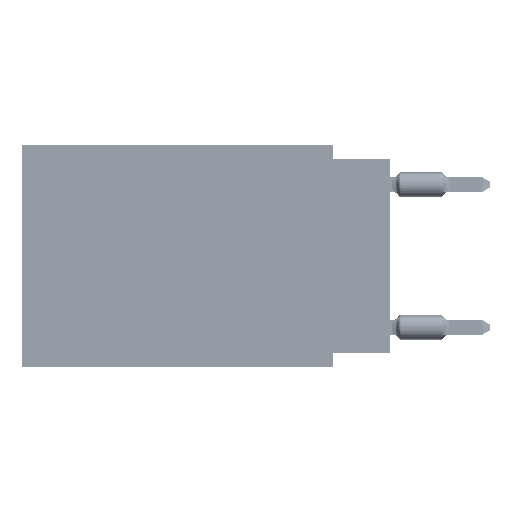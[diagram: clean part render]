
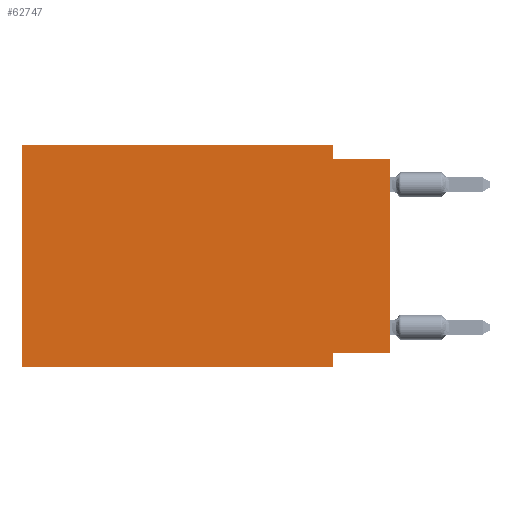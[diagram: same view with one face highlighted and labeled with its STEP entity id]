
A CAD part, left-side view. The second image highlights one B-rep face of the part: STEP entity #62747.
In plain terms, the highlighted planar face has unit normal (-1, 0, 0).
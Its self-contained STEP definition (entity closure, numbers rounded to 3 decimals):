
#709 = DIRECTION ( 'NONE',  ( 0., 0., -1. ) ) ;
#745 = LINE ( 'NONE', #27588, #38852 ) ;
#2618 = LINE ( 'NONE', #15208, #77627 ) ;
#3308 = EDGE_CURVE ( 'NONE', #63452, #78809, #53112, .T. ) ;
#4547 = VERTEX_POINT ( 'NONE', #11266 ) ;
#5590 = CARTESIAN_POINT ( 'NONE',  ( 0., 2.54, -9.271 ) ) ;
#5610 = EDGE_CURVE ( 'NONE', #64251, #78809, #2618, .T. ) ;
#5797 = VECTOR ( 'NONE', #46315, 1000. ) ;
#5839 = VERTEX_POINT ( 'NONE', #65967 ) ;
#6373 = VECTOR ( 'NONE', #71645, 1000. ) ;
#7146 = CARTESIAN_POINT ( 'NONE',  ( 0., 0., -0.635 ) ) ;
#11266 = CARTESIAN_POINT ( 'NONE',  ( 0., 2.54, -0.635 ) ) ;
#14900 = CARTESIAN_POINT ( 'NONE',  ( 0., 0., 0. ) ) ;
#15208 = CARTESIAN_POINT ( 'NONE',  ( 0., 16.383, -9.906 ) ) ;
#16245 = EDGE_CURVE ( 'NONE', #64251, #56325, #36313, .T. ) ;
#16995 = ORIENTED_EDGE ( 'NONE', *, *, #64843, .F. ) ;
#17209 = CARTESIAN_POINT ( 'NONE',  ( 0., 0., -9.271 ) ) ;
#17852 = EDGE_CURVE ( 'NONE', #73377, #50432, #28324, .T. ) ;
#22218 = EDGE_CURVE ( 'NONE', #56325, #5839, #745, .T. ) ;
#25203 = LINE ( 'NONE', #7146, #30240 ) ;
#26218 = CARTESIAN_POINT ( 'NONE',  ( 0., 2.54, -9.906 ) ) ;
#26559 = CARTESIAN_POINT ( 'NONE',  ( 0., 2.54, 0. ) ) ;
#27588 = CARTESIAN_POINT ( 'NONE',  ( 0., 16.383, 0. ) ) ;
#27906 = CARTESIAN_POINT ( 'NONE',  ( 0., 2.54, -9.906 ) ) ;
#28324 = LINE ( 'NONE', #14900, #6373 ) ;
#30240 = VECTOR ( 'NONE', #71432, 1000. ) ;
#30448 = ORIENTED_EDGE ( 'NONE', *, *, #17852, .T. ) ;
#32118 = DIRECTION ( 'NONE',  ( 0., 0., -1. ) ) ;
#33128 = VECTOR ( 'NONE', #32118, 1000. ) ;
#35963 = ORIENTED_EDGE ( 'NONE', *, *, #22218, .F. ) ;
#36313 = LINE ( 'NONE', #61942, #62507 ) ;
#38852 = VECTOR ( 'NONE', #52424, 1000. ) ;
#39352 = PLANE ( 'NONE',  #47727 ) ;
#39764 = DIRECTION ( 'NONE',  ( 1., 0., 0. ) ) ;
#42079 = DIRECTION ( 'NONE',  ( 0., -1., 0. ) ) ;
#42812 = EDGE_CURVE ( 'NONE', #73377, #63452, #69259, .T. ) ;
#43102 = ORIENTED_EDGE ( 'NONE', *, *, #82958, .F. ) ;
#43767 = ORIENTED_EDGE ( 'NONE', *, *, #42812, .F. ) ;
#45372 = ORIENTED_EDGE ( 'NONE', *, *, #3308, .F. ) ;
#46315 = DIRECTION ( 'NONE',  ( 0., 0., -1. ) ) ;
#47727 = AXIS2_PLACEMENT_3D ( 'NONE', #72121, #39764, #709 ) ;
#49108 = DIRECTION ( 'NONE',  ( 0., 1., 0. ) ) ;
#49828 = CARTESIAN_POINT ( 'NONE',  ( 0., 16.383, -9.906 ) ) ;
#50432 = VERTEX_POINT ( 'NONE', #71494 ) ;
#51837 = EDGE_LOOP ( 'NONE', ( #30448, #43102, #16995, #35963, #68385, #62359, #45372, #43767 ) ) ;
#52424 = DIRECTION ( 'NONE',  ( 0., -1., 0. ) ) ;
#53112 = LINE ( 'NONE', #26218, #33128 ) ;
#55994 = CARTESIAN_POINT ( 'NONE',  ( 0., 16.383, 0. ) ) ;
#56325 = VERTEX_POINT ( 'NONE', #55994 ) ;
#56646 = CARTESIAN_POINT ( 'NONE',  ( 0., 0., -9.271 ) ) ;
#61942 = CARTESIAN_POINT ( 'NONE',  ( 0., 16.383, 0. ) ) ;
#62359 = ORIENTED_EDGE ( 'NONE', *, *, #5610, .T. ) ;
#62507 = VECTOR ( 'NONE', #81264, 1000. ) ;
#62747 = ADVANCED_FACE ( 'NONE', ( #70883 ), #39352, .F. ) ;
#63452 = VERTEX_POINT ( 'NONE', #5590 ) ;
#64251 = VERTEX_POINT ( 'NONE', #49828 ) ;
#64811 = LINE ( 'NONE', #26559, #5797 ) ;
#64843 = EDGE_CURVE ( 'NONE', #5839, #4547, #64811, .T. ) ;
#65929 = VECTOR ( 'NONE', #49108, 1000. ) ;
#65967 = CARTESIAN_POINT ( 'NONE',  ( 0., 2.54, 0. ) ) ;
#68385 = ORIENTED_EDGE ( 'NONE', *, *, #16245, .F. ) ;
#69259 = LINE ( 'NONE', #56646, #65929 ) ;
#70883 = FACE_OUTER_BOUND ( 'NONE', #51837, .T. ) ;
#71432 = DIRECTION ( 'NONE',  ( 0., -1., 0. ) ) ;
#71494 = CARTESIAN_POINT ( 'NONE',  ( 0., 0., -0.635 ) ) ;
#71645 = DIRECTION ( 'NONE',  ( 0., 0., 1. ) ) ;
#72121 = CARTESIAN_POINT ( 'NONE',  ( 0., 16.383, 0. ) ) ;
#73377 = VERTEX_POINT ( 'NONE', #17209 ) ;
#77627 = VECTOR ( 'NONE', #42079, 1000. ) ;
#78809 = VERTEX_POINT ( 'NONE', #27906 ) ;
#81264 = DIRECTION ( 'NONE',  ( 0., 0., 1. ) ) ;
#82958 = EDGE_CURVE ( 'NONE', #4547, #50432, #25203, .T. ) ;
